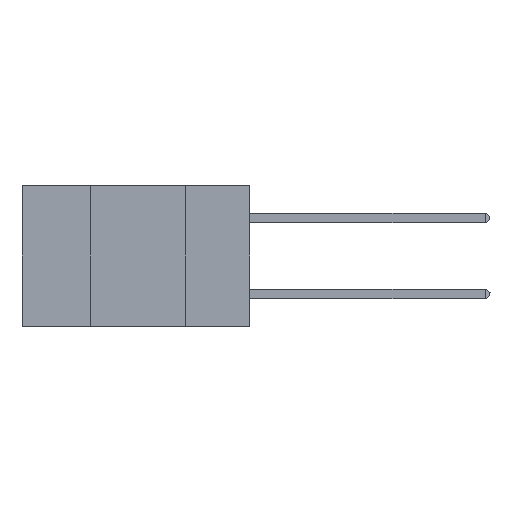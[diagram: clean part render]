
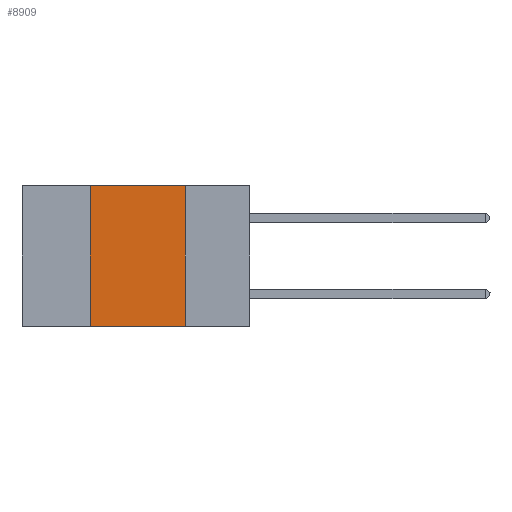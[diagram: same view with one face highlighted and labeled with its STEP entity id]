
A CAD part, left-side view. The second image highlights one B-rep face of the part: STEP entity #8909.
In plain terms, the highlighted planar face has unit normal (-1, 0, 0).
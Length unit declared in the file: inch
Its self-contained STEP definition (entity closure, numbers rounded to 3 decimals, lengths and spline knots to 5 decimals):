
#1762 = ORIENTED_EDGE ( 'NONE', *, *, #16678, .F. ) ;
#1971 = LINE ( 'NONE', #14126, #23093 ) ;
#2032 = EDGE_CURVE ( 'NONE', #6735, #6084, #16485, .T. ) ;
#2702 = DIRECTION ( 'NONE',  ( 0., -1., 0. ) ) ;
#3068 = EDGE_CURVE ( 'NONE', #6735, #11767, #12329, .T. ) ;
#3763 = DIRECTION ( 'NONE',  ( 0., 0., -1. ) ) ;
#4342 = VECTOR ( 'NONE', #23117, 39.37008 ) ;
#4710 = FACE_OUTER_BOUND ( 'NONE', #14297, .T. ) ;
#6084 = VERTEX_POINT ( 'NONE', #9496 ) ;
#6735 = VERTEX_POINT ( 'NONE', #26103 ) ;
#7214 = LINE ( 'NONE', #24922, #4342 ) ;
#7362 = CARTESIAN_POINT ( 'NONE',  ( 0., 0.17, 0. ) ) ;
#7620 = AXIS2_PLACEMENT_3D ( 'NONE', #11414, #25796, #25619 ) ;
#8909 = ADVANCED_FACE ( 'NONE', ( #4710 ), #19248, .F. ) ;
#9496 = CARTESIAN_POINT ( 'NONE',  ( 0., 0.42, 0. ) ) ;
#9771 = VECTOR ( 'NONE', #2702, 39.37008 ) ;
#10669 = CARTESIAN_POINT ( 'NONE',  ( 0., 0.17, -0.37 ) ) ;
#11414 = CARTESIAN_POINT ( 'NONE',  ( 0., 0.6, 0. ) ) ;
#11767 = VERTEX_POINT ( 'NONE', #10669 ) ;
#12329 = LINE ( 'NONE', #12989, #9771 ) ;
#12632 = VERTEX_POINT ( 'NONE', #7362 ) ;
#12989 = CARTESIAN_POINT ( 'NONE',  ( 0., 0.6, -0.37 ) ) ;
#13259 = VECTOR ( 'NONE', #25950, 39.37008 ) ;
#14126 = CARTESIAN_POINT ( 'NONE',  ( 0., 0.17, 0. ) ) ;
#14297 = EDGE_LOOP ( 'NONE', ( #1762, #21595, #18882, #24159 ) ) ;
#16485 = LINE ( 'NONE', #24157, #13259 ) ;
#16678 = EDGE_CURVE ( 'NONE', #12632, #11767, #1971, .T. ) ;
#18882 = ORIENTED_EDGE ( 'NONE', *, *, #2032, .F. ) ;
#19248 = PLANE ( 'NONE',  #7620 ) ;
#21595 = ORIENTED_EDGE ( 'NONE', *, *, #22392, .F. ) ;
#22392 = EDGE_CURVE ( 'NONE', #6084, #12632, #7214, .T. ) ;
#23093 = VECTOR ( 'NONE', #3763, 39.37008 ) ;
#23117 = DIRECTION ( 'NONE',  ( 0., -1., 0. ) ) ;
#24157 = CARTESIAN_POINT ( 'NONE',  ( 0., 0.42, 0. ) ) ;
#24159 = ORIENTED_EDGE ( 'NONE', *, *, #3068, .T. ) ;
#24922 = CARTESIAN_POINT ( 'NONE',  ( 0., 0.6, 0. ) ) ;
#25619 = DIRECTION ( 'NONE',  ( 0., 0., -1. ) ) ;
#25796 = DIRECTION ( 'NONE',  ( 1., 0., 0. ) ) ;
#25950 = DIRECTION ( 'NONE',  ( 0., 0., 1. ) ) ;
#26103 = CARTESIAN_POINT ( 'NONE',  ( 0., 0.42, -0.37 ) ) ;
